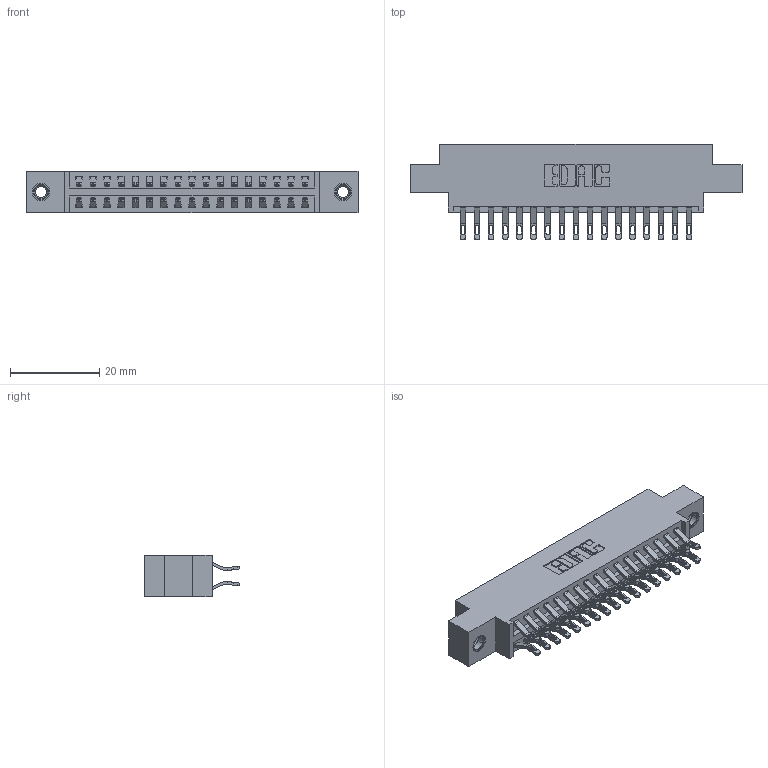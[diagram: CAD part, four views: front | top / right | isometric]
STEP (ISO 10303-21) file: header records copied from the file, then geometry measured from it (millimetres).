
FILE_DESCRIPTION (( 'STEP AP203' ), '1' );
FILE_NAME ('346-034-555-807.STEP', '2018-08-23T22:57:23', ( '' ), ( '' ), 'SwSTEP 2.0', 'SolidWorks 2016', '' );
FILE_SCHEMA (( 'CONFIG_CONTROL_DESIGN' ));
Length unit declared in the file: inch
Products named in the file (4): 346 Part_0.170 Offset - 0.156 Dia-TI; 345-292-001_555 Tail; 345-250-001_345-250-005-103; 346-034-555-807
Assembly tree (37 placements, depth 2):
  346-034-555-807
    346 Part_0.170 Offset - 0.156 Dia-TI
    345-292-001_555 Tail  x34
    345-250-001_345-250-005-103  x2
Bounding box: 74.55 x 21.46 x 9.4 mm (x, y, z)
Volume: 7005.8 mm3; surface area: 9801.9 mm2
Topology: 37 solids, 37 shells, 2158 faces, 6699 edges, 4458 vertices
Faces by surface type: plane 1234, cylinder 908, cone 12, torus 4
Entity records: 16104 total; most frequent: CARTESIAN_POINT 2709, ORIENTED_EDGE 2606, DIRECTION 2433, EDGE_CURVE 1303, LINE 1063, VECTOR 1063, VERTEX_POINT 864, AXIS2_PLACEMENT_3D 685
